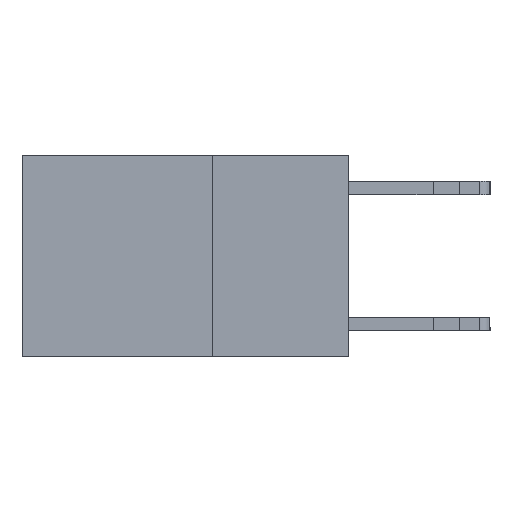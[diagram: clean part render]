
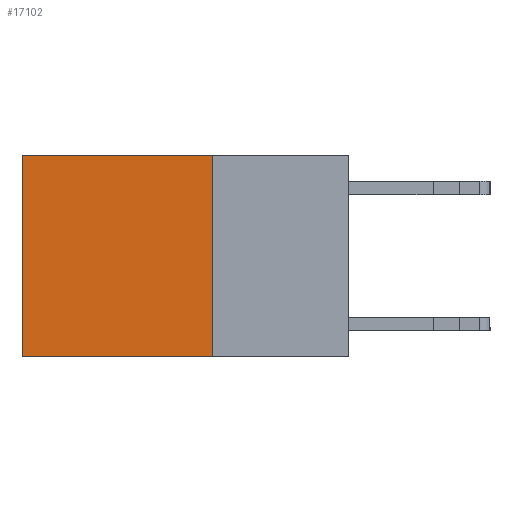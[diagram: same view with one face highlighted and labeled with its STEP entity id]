
A CAD part, left-side view. The second image highlights one B-rep face of the part: STEP entity #17102.
In plain terms, the highlighted planar face has unit normal (-1, 0, 0).
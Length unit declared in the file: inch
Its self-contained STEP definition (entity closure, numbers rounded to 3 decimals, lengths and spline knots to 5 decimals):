
#175 = VECTOR ( 'NONE', #19424, 39.37008 ) ;
#360 = EDGE_CURVE ( 'NONE', #23073, #4587, #4140, .T. ) ;
#1313 = ORIENTED_EDGE ( 'NONE', *, *, #4553, .T. ) ;
#1563 = CARTESIAN_POINT ( 'NONE',  ( 0.2625, 0.25, 0. ) ) ;
#2191 = CARTESIAN_POINT ( 'NONE',  ( 0.2625, 0.25, -0.37 ) ) ;
#2871 = DIRECTION ( 'NONE',  ( 0., 0., -1. ) ) ;
#3842 = EDGE_LOOP ( 'NONE', ( #1313, #9099, #5198, #24398 ) ) ;
#4140 = LINE ( 'NONE', #2191, #25534 ) ;
#4553 = EDGE_CURVE ( 'NONE', #13520, #4587, #12977, .T. ) ;
#4562 = FACE_OUTER_BOUND ( 'NONE', #3842, .T. ) ;
#4587 = VERTEX_POINT ( 'NONE', #21766 ) ;
#5198 = ORIENTED_EDGE ( 'NONE', *, *, #12452, .F. ) ;
#5491 = LINE ( 'NONE', #1563, #6581 ) ;
#6581 = VECTOR ( 'NONE', #18050, 39.37008 ) ;
#6836 = CARTESIAN_POINT ( 'NONE',  ( 0.2625, 0.25, -0.37 ) ) ;
#8385 = CARTESIAN_POINT ( 'NONE',  ( 0.2625, 0.6, 0. ) ) ;
#8630 = PLANE ( 'NONE',  #19371 ) ;
#9099 = ORIENTED_EDGE ( 'NONE', *, *, #360, .F. ) ;
#10170 = DIRECTION ( 'NONE',  ( 0., 1., 0. ) ) ;
#12151 = CARTESIAN_POINT ( 'NONE',  ( 0.2625, 0.25, 0. ) ) ;
#12452 = EDGE_CURVE ( 'NONE', #21927, #23073, #5491, .T. ) ;
#12977 = LINE ( 'NONE', #21127, #175 ) ;
#13520 = VERTEX_POINT ( 'NONE', #8385 ) ;
#14374 = VECTOR ( 'NONE', #15410, 39.37008 ) ;
#15410 = DIRECTION ( 'NONE',  ( 0., 1., 0. ) ) ;
#16361 = CARTESIAN_POINT ( 'NONE',  ( 0.2625, 0.25, 0. ) ) ;
#16488 = DIRECTION ( 'NONE',  ( 1., 0., 0. ) ) ;
#17102 = ADVANCED_FACE ( 'NONE', ( #4562 ), #8630, .F. ) ;
#17716 = EDGE_CURVE ( 'NONE', #21927, #13520, #18944, .T. ) ;
#18050 = DIRECTION ( 'NONE',  ( 0., 0., -1. ) ) ;
#18944 = LINE ( 'NONE', #22994, #14374 ) ;
#19371 = AXIS2_PLACEMENT_3D ( 'NONE', #16361, #16488, #2871 ) ;
#19424 = DIRECTION ( 'NONE',  ( 0., 0., -1. ) ) ;
#21127 = CARTESIAN_POINT ( 'NONE',  ( 0.2625, 0.6, 0. ) ) ;
#21766 = CARTESIAN_POINT ( 'NONE',  ( 0.2625, 0.6, -0.37 ) ) ;
#21927 = VERTEX_POINT ( 'NONE', #12151 ) ;
#22994 = CARTESIAN_POINT ( 'NONE',  ( 0.2625, 0.25, 0. ) ) ;
#23073 = VERTEX_POINT ( 'NONE', #6836 ) ;
#24398 = ORIENTED_EDGE ( 'NONE', *, *, #17716, .T. ) ;
#25534 = VECTOR ( 'NONE', #10170, 39.37008 ) ;
